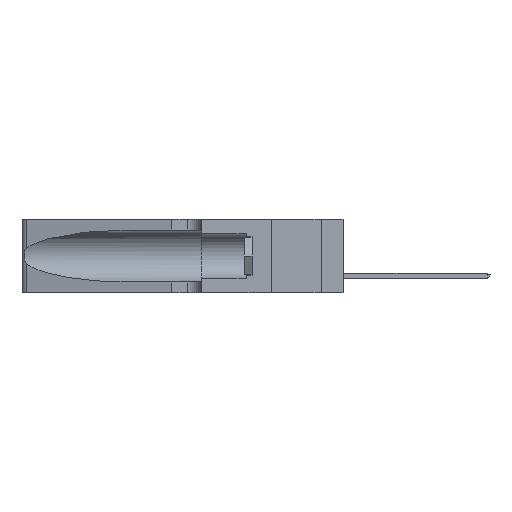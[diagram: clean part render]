
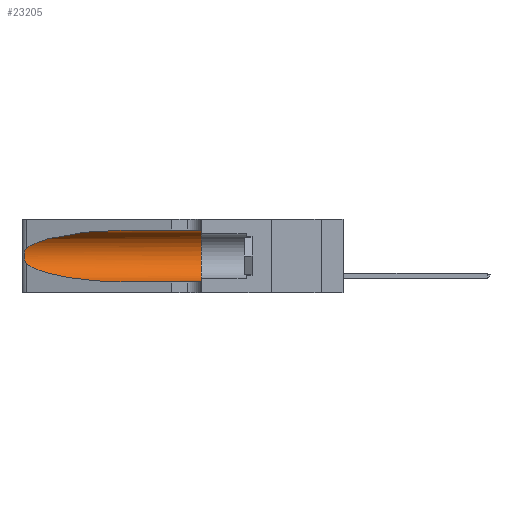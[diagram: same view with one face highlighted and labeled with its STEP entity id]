
A CAD part, left-side view. The second image highlights one B-rep face of the part: STEP entity #23205.
In plain terms, the highlighted cylindrical face has radius 3.308 mm (diameter 6.617 mm), a partial arc.
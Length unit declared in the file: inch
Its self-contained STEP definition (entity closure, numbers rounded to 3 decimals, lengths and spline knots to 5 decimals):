
#96 = DIRECTION ( 'NONE',  ( 0., -1., 0. ) ) ;
#403 = ORIENTED_EDGE ( 'NONE', *, *, #14164, .T. ) ;
#479 = CARTESIAN_POINT ( 'NONE',  ( 0.1305, 0.72297, 0.31525 ) ) ;
#644 = CARTESIAN_POINT ( 'NONE',  ( 0.18966, 0.96281, 0.31525 ) ) ;
#797 =( BOUNDED_CURVE ( )  B_SPLINE_CURVE ( 3, ( #11349, #18621, #11034, #22337 ),
 .UNSPECIFIED., .F., .T. ) 
 B_SPLINE_CURVE_WITH_KNOTS ( ( 4, 4 ),
 ( 3.44316, 4.71239 ),
 .UNSPECIFIED. ) 
 CURVE ( )  GEOMETRIC_REPRESENTATION_ITEM ( )  RATIONAL_B_SPLINE_CURVE ( ( 1., 0.87, 0.87, 1. ) ) 
 REPRESENTATION_ITEM ( '' )  );
#1258 = VERTEX_POINT ( 'NONE', #22059 ) ;
#1795 = CYLINDRICAL_SURFACE ( 'NONE', #16363, 0.13025 ) ;
#2302 = CARTESIAN_POINT ( 'NONE',  ( 0.1305, 0.35, 0.185 ) ) ;
#3456 = CARTESIAN_POINT ( 'NONE',  ( 0.1305, 1.61858, 0.05475 ) ) ;
#3530 = DIRECTION ( 'NONE',  ( 0., -1., 0. ) ) ;
#3781 = VECTOR ( 'NONE', #3530, 39.37008 ) ;
#3849 = CARTESIAN_POINT ( 'NONE',  ( 0.25487, 1.22718, 0.22369 ) ) ;
#3920 = DIRECTION ( 'NONE',  ( 0., 1., 0. ) ) ;
#4962 = ORIENTED_EDGE ( 'NONE', *, *, #16883, .T. ) ;
#5176 = DIRECTION ( 'NONE',  ( 0., -1., 0. ) ) ;
#6602 = CARTESIAN_POINT ( 'NONE',  ( 0.2373, 1.15595, 0.28018 ) ) ;
#7098 = CARTESIAN_POINT ( 'NONE',  ( 0.1305, 1.61858, 0.31525 ) ) ;
#7105 = CARTESIAN_POINT ( 'NONE',  ( 0.25555, 1.22993, 0.14849 ) ) ;
#7406 = CARTESIAN_POINT ( 'NONE',  ( 0.25787, 1.23484, 0.2124 ) ) ;
#7486 = VERTEX_POINT ( 'NONE', #3849 ) ;
#7588 = ORIENTED_EDGE ( 'NONE', *, *, #11456, .T. ) ;
#8823 = LINE ( 'NONE', #7098, #10826 ) ;
#8940 = CARTESIAN_POINT ( 'NONE',  ( 0.25487, 1.22718, 0.14631 ) ) ;
#10714 = CARTESIAN_POINT ( 'NONE',  ( 0.26018, 1.23835, 0.19895 ) ) ;
#10826 = VECTOR ( 'NONE', #5176, 39.37008 ) ;
#11011 = CARTESIAN_POINT ( 'NONE',  ( 0.25555, 1.22994, 0.2215 ) ) ;
#11034 = CARTESIAN_POINT ( 'NONE',  ( 0.18966, 0.96281, 0.05475 ) ) ;
#11168 = DIRECTION ( 'NONE',  ( 0., 0., -1. ) ) ;
#11275 = FACE_OUTER_BOUND ( 'NONE', #20215, .T. ) ;
#11349 = CARTESIAN_POINT ( 'NONE',  ( 0.25487, 1.22718, 0.14631 ) ) ;
#11456 = EDGE_CURVE ( 'NONE', #15560, #11553, #797, .T. ) ;
#11553 = VERTEX_POINT ( 'NONE', #16516 ) ;
#11823 =( BOUNDED_CURVE ( )  B_SPLINE_CURVE ( 3, ( #22676, #644, #6602, #23185 ),
 .UNSPECIFIED., .F., .F. ) 
 B_SPLINE_CURVE_WITH_KNOTS ( ( 4, 4 ),
 ( 1.5708, 2.84003 ),
 .UNSPECIFIED. ) 
 CURVE ( )  GEOMETRIC_REPRESENTATION_ITEM ( )  RATIONAL_B_SPLINE_CURVE ( ( 1., 0.87, 0.87, 1. ) ) 
 REPRESENTATION_ITEM ( '' )  );
#12094 = LINE ( 'NONE', #3456, #3781 ) ;
#12419 = AXIS2_PLACEMENT_3D ( 'NONE', #2302, #3920, #18945 ) ;
#12540 = CARTESIAN_POINT ( 'NONE',  ( 0.26075, 1.23896, 0.178 ) ) ;
#12676 = ORIENTED_EDGE ( 'NONE', *, *, #20269, .F. ) ;
#12698 = CARTESIAN_POINT ( 'NONE',  ( 0.25639, 1.23186, 0.15144 ) ) ;
#12773 = VERTEX_POINT ( 'NONE', #479 ) ;
#12860 = CARTESIAN_POINT ( 'NONE',  ( 0.1305, 1.61858, 0.185 ) ) ;
#13542 = CARTESIAN_POINT ( 'NONE',  ( 0.25487, 1.22718, 0.14631 ) ) ;
#13797 = CIRCLE ( 'NONE', #12419, 0.13025 ) ;
#14164 = EDGE_CURVE ( 'NONE', #7486, #15560, #16124, .T. ) ;
#14358 = ORIENTED_EDGE ( 'NONE', *, *, #16348, .F. ) ;
#14510 = CARTESIAN_POINT ( 'NONE',  ( 0.26017, 1.23833, 0.17102 ) ) ;
#15560 = VERTEX_POINT ( 'NONE', #13542 ) ;
#16124 = B_SPLINE_CURVE_WITH_KNOTS ( 'NONE', 3,
 ( #23615, #11011, #18276, #7406, #20289, #10714, #21824, #12540, #14510, #18112, #21912, #12698, #7105, #8940 ),
 .UNSPECIFIED., .F., .F.,
 ( 4, 2, 2, 2, 2, 2, 4 ),
 ( 0., 0.00027, 0.00053, 0.00107, 0.0016, 0.00187, 0.00214 ),
 .UNSPECIFIED. ) ;
#16348 = EDGE_CURVE ( 'NONE', #12773, #18041, #8823, .T. ) ;
#16363 = AXIS2_PLACEMENT_3D ( 'NONE', #12860, #96, #11168 ) ;
#16516 = CARTESIAN_POINT ( 'NONE',  ( 0.1305, 0.72297, 0.05475 ) ) ;
#16883 = EDGE_CURVE ( 'NONE', #12773, #7486, #11823, .T. ) ;
#17875 = ORIENTED_EDGE ( 'NONE', *, *, #23729, .T. ) ;
#18041 = VERTEX_POINT ( 'NONE', #21264 ) ;
#18112 = CARTESIAN_POINT ( 'NONE',  ( 0.25856, 1.23593, 0.16098 ) ) ;
#18276 = CARTESIAN_POINT ( 'NONE',  ( 0.25639, 1.23184, 0.21858 ) ) ;
#18621 = CARTESIAN_POINT ( 'NONE',  ( 0.2373, 1.15595, 0.08982 ) ) ;
#18945 = DIRECTION ( 'NONE',  ( 0., 0., 1. ) ) ;
#20215 = EDGE_LOOP ( 'NONE', ( #4962, #403, #7588, #17875, #12676, #14358 ) ) ;
#20269 = EDGE_CURVE ( 'NONE', #18041, #1258, #13797, .T. ) ;
#20289 = CARTESIAN_POINT ( 'NONE',  ( 0.25854, 1.2359, 0.20912 ) ) ;
#21264 = CARTESIAN_POINT ( 'NONE',  ( 0.1305, 0.35, 0.31525 ) ) ;
#21824 = CARTESIAN_POINT ( 'NONE',  ( 0.26075, 1.23896, 0.19203 ) ) ;
#21912 = CARTESIAN_POINT ( 'NONE',  ( 0.25789, 1.23486, 0.15765 ) ) ;
#22059 = CARTESIAN_POINT ( 'NONE',  ( 0.1305, 0.35, 0.05475 ) ) ;
#22337 = CARTESIAN_POINT ( 'NONE',  ( 0.1305, 0.72297, 0.05475 ) ) ;
#22676 = CARTESIAN_POINT ( 'NONE',  ( 0.1305, 0.72297, 0.31525 ) ) ;
#23185 = CARTESIAN_POINT ( 'NONE',  ( 0.25487, 1.22718, 0.22369 ) ) ;
#23205 = ADVANCED_FACE ( 'NONE', ( #11275 ), #1795, .F. ) ;
#23615 = CARTESIAN_POINT ( 'NONE',  ( 0.25487, 1.22718, 0.22369 ) ) ;
#23729 = EDGE_CURVE ( 'NONE', #11553, #1258, #12094, .T. ) ;
